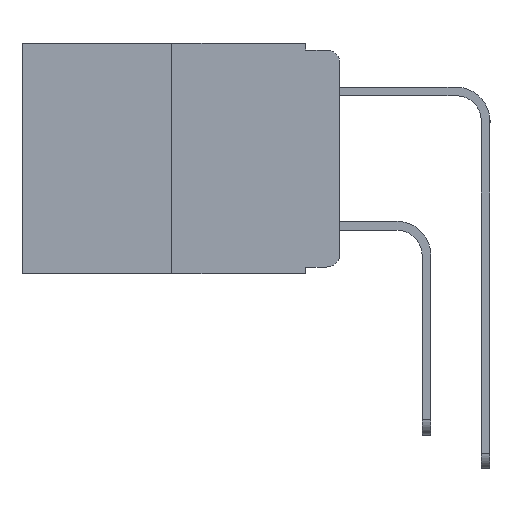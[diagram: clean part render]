
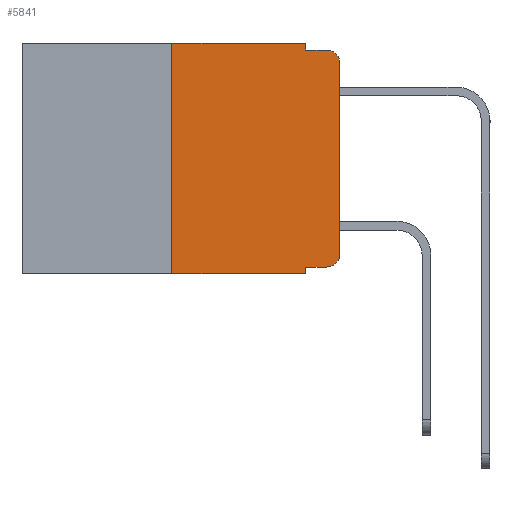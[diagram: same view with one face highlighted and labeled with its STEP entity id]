
A CAD part, left-side view. The second image highlights one B-rep face of the part: STEP entity #5841.
In plain terms, the highlighted planar face has unit normal (-1, 0, 0).
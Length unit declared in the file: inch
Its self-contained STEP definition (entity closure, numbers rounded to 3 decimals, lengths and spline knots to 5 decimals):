
#69 = VERTEX_POINT ( 'NONE', #15736 ) ;
#265 = CIRCLE ( 'NONE', #14807, 0.02 ) ;
#286 = CARTESIAN_POINT ( 'NONE',  ( 0., 0.02, -0.333 ) ) ;
#381 = CARTESIAN_POINT ( 'NONE',  ( 0., 0.051, -0.333 ) ) ;
#503 = ORIENTED_EDGE ( 'NONE', *, *, #8614, .F. ) ;
#607 = CARTESIAN_POINT ( 'NONE',  ( 0., 0.051, 0. ) ) ;
#646 = CARTESIAN_POINT ( 'NONE',  ( 0., 0.02, -0.03 ) ) ;
#1161 = ORIENTED_EDGE ( 'NONE', *, *, #18093, .F. ) ;
#1397 = VERTEX_POINT ( 'NONE', #607 ) ;
#1560 = DIRECTION ( 'NONE',  ( 0., -1., 0. ) ) ;
#1873 = CARTESIAN_POINT ( 'NONE',  ( 0., 0.473, 0. ) ) ;
#1932 = ORIENTED_EDGE ( 'NONE', *, *, #9595, .F. ) ;
#2244 = DIRECTION ( 'NONE',  ( 0., 0., -1. ) ) ;
#2556 = CARTESIAN_POINT ( 'NONE',  ( 0., 0.051, 0. ) ) ;
#2913 = CARTESIAN_POINT ( 'NONE',  ( 0., 0.25, -0.343 ) ) ;
#3121 = LINE ( 'NONE', #13637, #6822 ) ;
#3359 = VERTEX_POINT ( 'NONE', #2913 ) ;
#4046 = DIRECTION ( 'NONE',  ( -1., 0., 0. ) ) ;
#4243 = DIRECTION ( 'NONE',  ( 0., 0., -1. ) ) ;
#4596 = EDGE_LOOP ( 'NONE', ( #16032, #5203, #15696, #6844, #1161, #1932, #14214, #503, #5843, #7259 ) ) ;
#5203 = ORIENTED_EDGE ( 'NONE', *, *, #13480, .T. ) ;
#5283 = VECTOR ( 'NONE', #6151, 39.37008 ) ;
#5841 = ADVANCED_FACE ( 'NONE', ( #12322 ), #11097, .F. ) ;
#5843 = ORIENTED_EDGE ( 'NONE', *, *, #7582, .T. ) ;
#5986 = VERTEX_POINT ( 'NONE', #10024 ) ;
#6007 = CARTESIAN_POINT ( 'NONE',  ( 0., 0.051, -0.343 ) ) ;
#6151 = DIRECTION ( 'NONE',  ( 0., -1., 0. ) ) ;
#6603 = EDGE_CURVE ( 'NONE', #13335, #8241, #265, .T. ) ;
#6822 = VECTOR ( 'NONE', #15062, 39.37008 ) ;
#6844 = ORIENTED_EDGE ( 'NONE', *, *, #10577, .F. ) ;
#6884 = CARTESIAN_POINT ( 'NONE',  ( 0., 0.051, -0.01 ) ) ;
#7157 = VECTOR ( 'NONE', #17848, 39.37008 ) ;
#7259 = ORIENTED_EDGE ( 'NONE', *, *, #6603, .T. ) ;
#7582 = EDGE_CURVE ( 'NONE', #11367, #13335, #18198, .T. ) ;
#7761 = CARTESIAN_POINT ( 'NONE',  ( 0., 0.051, -0.333 ) ) ;
#7817 = LINE ( 'NONE', #2556, #11259 ) ;
#7891 = DIRECTION ( 'NONE',  ( 0., 0., -1. ) ) ;
#8224 = DIRECTION ( 'NONE',  ( 1., 0., 0. ) ) ;
#8241 = VERTEX_POINT ( 'NONE', #10775 ) ;
#8614 = EDGE_CURVE ( 'NONE', #11367, #14285, #7817, .T. ) ;
#8729 = AXIS2_PLACEMENT_3D ( 'NONE', #646, #11424, #2244 ) ;
#8884 = CARTESIAN_POINT ( 'NONE',  ( 0., 0., -0.03 ) ) ;
#9004 = CARTESIAN_POINT ( 'NONE',  ( 0., 0.25, 0. ) ) ;
#9379 = CARTESIAN_POINT ( 'NONE',  ( 0., 0.473, -0.343 ) ) ;
#9595 = EDGE_CURVE ( 'NONE', #3359, #5986, #13538, .T. ) ;
#10024 = CARTESIAN_POINT ( 'NONE',  ( 0., 0.25, 0. ) ) ;
#10566 = VECTOR ( 'NONE', #7891, 39.37008 ) ;
#10577 = EDGE_CURVE ( 'NONE', #1397, #11445, #14391, .T. ) ;
#10775 = CARTESIAN_POINT ( 'NONE',  ( 0., 0., -0.313 ) ) ;
#10790 = CARTESIAN_POINT ( 'NONE',  ( 0., 0.051, 0. ) ) ;
#11097 = PLANE ( 'NONE',  #17388 ) ;
#11259 = VECTOR ( 'NONE', #4243, 39.37008 ) ;
#11367 = VERTEX_POINT ( 'NONE', #381 ) ;
#11424 = DIRECTION ( 'NONE',  ( -1., 0., 0. ) ) ;
#11445 = VERTEX_POINT ( 'NONE', #6884 ) ;
#11786 = LINE ( 'NONE', #9379, #19326 ) ;
#12259 = CIRCLE ( 'NONE', #8729, 0.02 ) ;
#12322 = FACE_OUTER_BOUND ( 'NONE', #4596, .T. ) ;
#12497 = EDGE_CURVE ( 'NONE', #11445, #69, #13217, .T. ) ;
#12749 = VECTOR ( 'NONE', #17997, 39.37008 ) ;
#12981 = CARTESIAN_POINT ( 'NONE',  ( 0., 0.02, -0.313 ) ) ;
#13217 = LINE ( 'NONE', #16597, #12749 ) ;
#13335 = VERTEX_POINT ( 'NONE', #286 ) ;
#13480 = EDGE_CURVE ( 'NONE', #18475, #69, #12259, .T. ) ;
#13538 = LINE ( 'NONE', #9004, #16838 ) ;
#13637 = CARTESIAN_POINT ( 'NONE',  ( 0., 0., 0. ) ) ;
#14214 = ORIENTED_EDGE ( 'NONE', *, *, #16906, .T. ) ;
#14285 = VERTEX_POINT ( 'NONE', #6007 ) ;
#14391 = LINE ( 'NONE', #10790, #10566 ) ;
#14422 = DIRECTION ( 'NONE',  ( 0., 0., -1. ) ) ;
#14432 = EDGE_CURVE ( 'NONE', #8241, #18475, #3121, .T. ) ;
#14720 = DIRECTION ( 'NONE',  ( 0., 0., 1. ) ) ;
#14807 = AXIS2_PLACEMENT_3D ( 'NONE', #12981, #4046, #14422 ) ;
#15062 = DIRECTION ( 'NONE',  ( 0., 0., 1. ) ) ;
#15696 = ORIENTED_EDGE ( 'NONE', *, *, #12497, .F. ) ;
#15736 = CARTESIAN_POINT ( 'NONE',  ( 0., 0.02, -0.01 ) ) ;
#16032 = ORIENTED_EDGE ( 'NONE', *, *, #14432, .T. ) ;
#16318 = CARTESIAN_POINT ( 'NONE',  ( 0., 0.473, 0. ) ) ;
#16597 = CARTESIAN_POINT ( 'NONE',  ( 0., 0.051, -0.01 ) ) ;
#16838 = VECTOR ( 'NONE', #14720, 39.37008 ) ;
#16897 = LINE ( 'NONE', #16318, #5283 ) ;
#16906 = EDGE_CURVE ( 'NONE', #3359, #14285, #11786, .T. ) ;
#17388 = AXIS2_PLACEMENT_3D ( 'NONE', #1873, #8224, #18246 ) ;
#17848 = DIRECTION ( 'NONE',  ( 0., -1., 0. ) ) ;
#17997 = DIRECTION ( 'NONE',  ( 0., -1., 0. ) ) ;
#18093 = EDGE_CURVE ( 'NONE', #5986, #1397, #16897, .T. ) ;
#18198 = LINE ( 'NONE', #7761, #7157 ) ;
#18246 = DIRECTION ( 'NONE',  ( 0., 0., -1. ) ) ;
#18475 = VERTEX_POINT ( 'NONE', #8884 ) ;
#19326 = VECTOR ( 'NONE', #1560, 39.37008 ) ;
